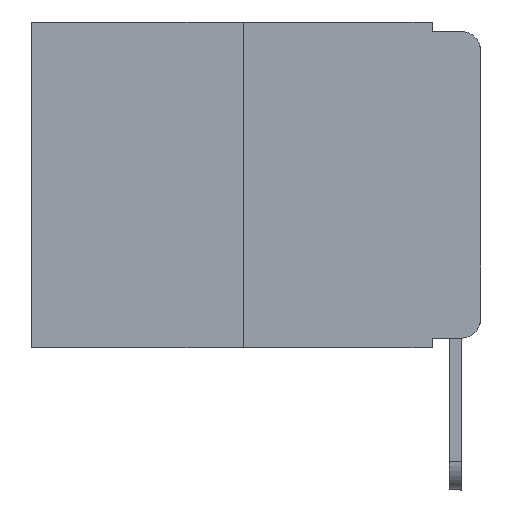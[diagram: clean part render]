
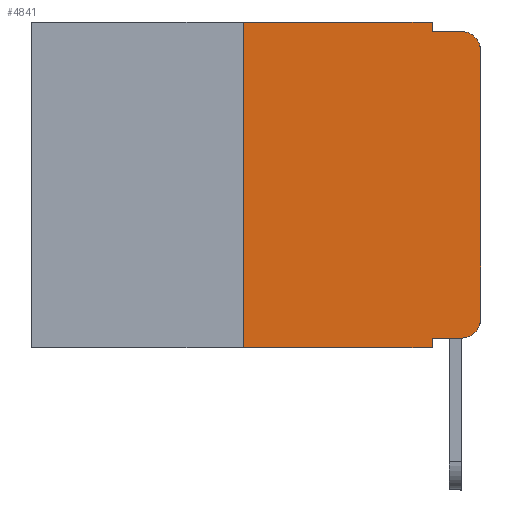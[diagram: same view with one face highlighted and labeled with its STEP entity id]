
A CAD part, left-side view. The second image highlights one B-rep face of the part: STEP entity #4841.
In plain terms, the highlighted planar face has unit normal (-1, 0, 0).
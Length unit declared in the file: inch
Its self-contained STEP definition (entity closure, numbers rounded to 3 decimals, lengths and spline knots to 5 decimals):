
#170 = VECTOR ( 'NONE', #13500, 39.37008 ) ;
#224 = EDGE_CURVE ( 'NONE', #16040, #20661, #13358, .T. ) ;
#471 = EDGE_CURVE ( 'NONE', #5555, #11577, #5261, .T. ) ;
#865 = ORIENTED_EDGE ( 'NONE', *, *, #15631, .F. ) ;
#897 = DIRECTION ( 'NONE',  ( -1., 0., 0. ) ) ;
#1270 = DIRECTION ( 'NONE',  ( 1., 0., 0. ) ) ;
#1602 = AXIS2_PLACEMENT_3D ( 'NONE', #6795, #897, #4664 ) ;
#2150 = LINE ( 'NONE', #13995, #11487 ) ;
#3095 = CARTESIAN_POINT ( 'NONE',  ( 0., 0.02, -0.333 ) ) ;
#3477 = EDGE_CURVE ( 'NONE', #17874, #11558, #11655, .T. ) ;
#3481 = LINE ( 'NONE', #19105, #13766 ) ;
#3548 = ORIENTED_EDGE ( 'NONE', *, *, #224, .F. ) ;
#3612 = ORIENTED_EDGE ( 'NONE', *, *, #17416, .T. ) ;
#4070 = DIRECTION ( 'NONE',  ( 0., 0., 1. ) ) ;
#4664 = DIRECTION ( 'NONE',  ( 0., 0., -1. ) ) ;
#4841 = ADVANCED_FACE ( 'NONE', ( #20663 ), #24572, .F. ) ;
#4877 = AXIS2_PLACEMENT_3D ( 'NONE', #18776, #1270, #14997 ) ;
#5097 = CIRCLE ( 'NONE', #12753, 0.02 ) ;
#5261 = LINE ( 'NONE', #18272, #15545 ) ;
#5267 = VECTOR ( 'NONE', #18443, 39.37008 ) ;
#5555 = VERTEX_POINT ( 'NONE', #12315 ) ;
#5630 = CARTESIAN_POINT ( 'NONE',  ( 0., 0.473, -0.343 ) ) ;
#5700 = LINE ( 'NONE', #7971, #13431 ) ;
#5786 = DIRECTION ( 'NONE',  ( 0., 0., -1. ) ) ;
#6259 = CARTESIAN_POINT ( 'NONE',  ( 0., 0.051, -0.333 ) ) ;
#6795 = CARTESIAN_POINT ( 'NONE',  ( 0., 0.02, -0.313 ) ) ;
#7091 = CARTESIAN_POINT ( 'NONE',  ( 0., 0., 0. ) ) ;
#7383 = DIRECTION ( 'NONE',  ( 0., -1., 0. ) ) ;
#7408 = ORIENTED_EDGE ( 'NONE', *, *, #24547, .F. ) ;
#7677 = VERTEX_POINT ( 'NONE', #12580 ) ;
#7971 = CARTESIAN_POINT ( 'NONE',  ( 0., 0.25, 0. ) ) ;
#8291 = VERTEX_POINT ( 'NONE', #14036 ) ;
#9054 = DIRECTION ( 'NONE',  ( 0., 0., -1. ) ) ;
#9681 = DIRECTION ( 'NONE',  ( 0., 0., -1. ) ) ;
#9798 = EDGE_LOOP ( 'NONE', ( #15449, #3612, #7408, #21976, #865, #10835, #18234, #3548, #21269, #24665 ) ) ;
#10219 = DIRECTION ( 'NONE',  ( 0., -1., 0. ) ) ;
#10835 = ORIENTED_EDGE ( 'NONE', *, *, #12824, .F. ) ;
#10985 = EDGE_CURVE ( 'NONE', #16040, #17874, #3481, .T. ) ;
#11228 = LINE ( 'NONE', #11729, #170 ) ;
#11487 = VECTOR ( 'NONE', #10219, 39.37008 ) ;
#11558 = VERTEX_POINT ( 'NONE', #21664 ) ;
#11577 = VERTEX_POINT ( 'NONE', #13873 ) ;
#11655 = CIRCLE ( 'NONE', #1602, 0.02 ) ;
#11729 = CARTESIAN_POINT ( 'NONE',  ( 0., 0.051, -0.01 ) ) ;
#12260 = CARTESIAN_POINT ( 'NONE',  ( 0., 0.02, -0.01 ) ) ;
#12315 = CARTESIAN_POINT ( 'NONE',  ( 0., 0.051, 0. ) ) ;
#12580 = CARTESIAN_POINT ( 'NONE',  ( 0., 0.25, -0.343 ) ) ;
#12600 = VERTEX_POINT ( 'NONE', #18582 ) ;
#12753 = AXIS2_PLACEMENT_3D ( 'NONE', #13971, #21641, #9681 ) ;
#12824 = EDGE_CURVE ( 'NONE', #7677, #8291, #5700, .T. ) ;
#13358 = LINE ( 'NONE', #19409, #16318 ) ;
#13431 = VECTOR ( 'NONE', #4070, 39.37008 ) ;
#13500 = DIRECTION ( 'NONE',  ( 0., -1., 0. ) ) ;
#13766 = VECTOR ( 'NONE', #7383, 39.37008 ) ;
#13817 = VECTOR ( 'NONE', #17110, 39.37008 ) ;
#13873 = CARTESIAN_POINT ( 'NONE',  ( 0., 0.051, -0.01 ) ) ;
#13971 = CARTESIAN_POINT ( 'NONE',  ( 0., 0.02, -0.03 ) ) ;
#13995 = CARTESIAN_POINT ( 'NONE',  ( 0., 0.473, 0. ) ) ;
#14036 = CARTESIAN_POINT ( 'NONE',  ( 0., 0.25, 0. ) ) ;
#14997 = DIRECTION ( 'NONE',  ( 0., 0., -1. ) ) ;
#15449 = ORIENTED_EDGE ( 'NONE', *, *, #20031, .T. ) ;
#15545 = VECTOR ( 'NONE', #9054, 39.37008 ) ;
#15631 = EDGE_CURVE ( 'NONE', #8291, #5555, #2150, .T. ) ;
#16040 = VERTEX_POINT ( 'NONE', #6259 ) ;
#16318 = VECTOR ( 'NONE', #5786, 39.37008 ) ;
#17110 = DIRECTION ( 'NONE',  ( 0., -1., 0. ) ) ;
#17135 = CARTESIAN_POINT ( 'NONE',  ( 0., 0.051, -0.343 ) ) ;
#17416 = EDGE_CURVE ( 'NONE', #12600, #20330, #5097, .T. ) ;
#17874 = VERTEX_POINT ( 'NONE', #3095 ) ;
#18234 = ORIENTED_EDGE ( 'NONE', *, *, #22384, .T. ) ;
#18272 = CARTESIAN_POINT ( 'NONE',  ( 0., 0.051, 0. ) ) ;
#18443 = DIRECTION ( 'NONE',  ( 0., 0., 1. ) ) ;
#18582 = CARTESIAN_POINT ( 'NONE',  ( 0., 0., -0.03 ) ) ;
#18776 = CARTESIAN_POINT ( 'NONE',  ( 0., 0.473, 0. ) ) ;
#19105 = CARTESIAN_POINT ( 'NONE',  ( 0., 0.051, -0.333 ) ) ;
#19409 = CARTESIAN_POINT ( 'NONE',  ( 0., 0.051, 0. ) ) ;
#20031 = EDGE_CURVE ( 'NONE', #11558, #12600, #22351, .T. ) ;
#20330 = VERTEX_POINT ( 'NONE', #12260 ) ;
#20661 = VERTEX_POINT ( 'NONE', #17135 ) ;
#20663 = FACE_OUTER_BOUND ( 'NONE', #9798, .T. ) ;
#21269 = ORIENTED_EDGE ( 'NONE', *, *, #10985, .T. ) ;
#21641 = DIRECTION ( 'NONE',  ( -1., 0., 0. ) ) ;
#21664 = CARTESIAN_POINT ( 'NONE',  ( 0., 0., -0.313 ) ) ;
#21976 = ORIENTED_EDGE ( 'NONE', *, *, #471, .F. ) ;
#22351 = LINE ( 'NONE', #7091, #5267 ) ;
#22384 = EDGE_CURVE ( 'NONE', #7677, #20661, #23287, .T. ) ;
#23287 = LINE ( 'NONE', #5630, #13817 ) ;
#24547 = EDGE_CURVE ( 'NONE', #11577, #20330, #11228, .T. ) ;
#24572 = PLANE ( 'NONE',  #4877 ) ;
#24665 = ORIENTED_EDGE ( 'NONE', *, *, #3477, .T. ) ;
